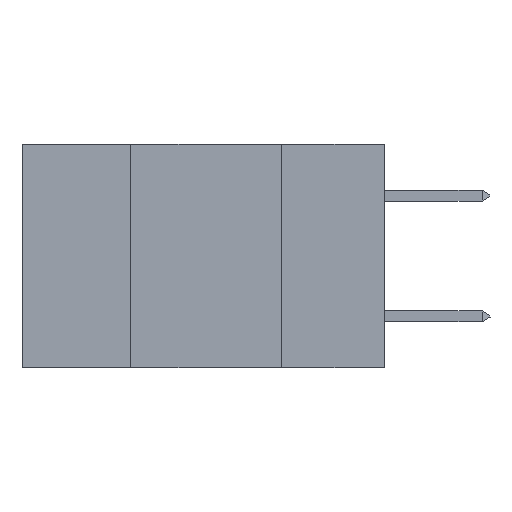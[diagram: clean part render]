
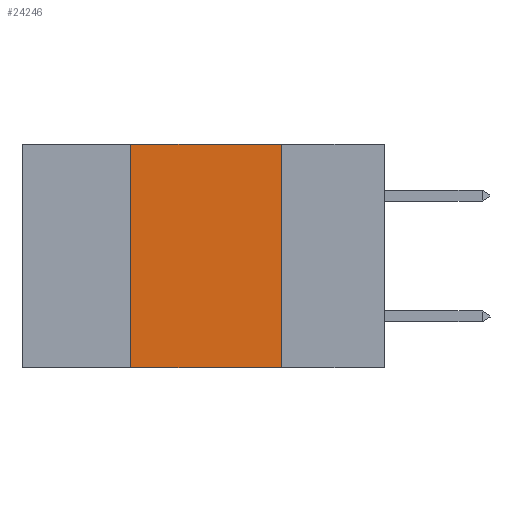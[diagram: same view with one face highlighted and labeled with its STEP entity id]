
A CAD part, left-side view. The second image highlights one B-rep face of the part: STEP entity #24246.
In plain terms, the highlighted planar face has unit normal (-1, 0, 0).
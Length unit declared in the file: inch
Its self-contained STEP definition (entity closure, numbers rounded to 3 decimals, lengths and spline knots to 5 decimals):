
#930 = ORIENTED_EDGE ( 'NONE', *, *, #37264, .F. ) ;
#1995 = DIRECTION ( 'NONE',  ( 0., 0., -1. ) ) ;
#4105 = DIRECTION ( 'NONE',  ( 0., -1., 0. ) ) ;
#5628 = CARTESIAN_POINT ( 'NONE',  ( 0., 0.17, -0.37 ) ) ;
#5698 = LINE ( 'NONE', #14263, #31536 ) ;
#7103 = EDGE_CURVE ( 'NONE', #25348, #16699, #5698, .T. ) ;
#7893 = ORIENTED_EDGE ( 'NONE', *, *, #35387, .F. ) ;
#10733 = DIRECTION ( 'NONE',  ( 0., -1., 0. ) ) ;
#10874 = CARTESIAN_POINT ( 'NONE',  ( 0., 0.17, 0. ) ) ;
#14263 = CARTESIAN_POINT ( 'NONE',  ( 0., 0.6, 0. ) ) ;
#15130 = PLANE ( 'NONE',  #18716 ) ;
#15509 = CARTESIAN_POINT ( 'NONE',  ( 0., 0.42, 0. ) ) ;
#16658 = EDGE_CURVE ( 'NONE', #29449, #40052, #29981, .T. ) ;
#16699 = VERTEX_POINT ( 'NONE', #10874 ) ;
#18544 = DIRECTION ( 'NONE',  ( 1., 0., 0. ) ) ;
#18716 = AXIS2_PLACEMENT_3D ( 'NONE', #35076, #18544, #41714 ) ;
#19047 = CARTESIAN_POINT ( 'NONE',  ( 0., 0.17, 0. ) ) ;
#19973 = LINE ( 'NONE', #19047, #27820 ) ;
#20650 = CARTESIAN_POINT ( 'NONE',  ( 0., 0.42, 0. ) ) ;
#21127 = VECTOR ( 'NONE', #10733, 39.37008 ) ;
#22186 = LINE ( 'NONE', #15509, #30266 ) ;
#24246 = ADVANCED_FACE ( 'NONE', ( #38545 ), #15130, .F. ) ;
#25348 = VERTEX_POINT ( 'NONE', #20650 ) ;
#26983 = CARTESIAN_POINT ( 'NONE',  ( 0., 0.6, -0.37 ) ) ;
#27155 = EDGE_LOOP ( 'NONE', ( #7893, #35723, #930, #37794 ) ) ;
#27820 = VECTOR ( 'NONE', #1995, 39.37008 ) ;
#28464 = CARTESIAN_POINT ( 'NONE',  ( 0., 0.42, -0.37 ) ) ;
#28834 = DIRECTION ( 'NONE',  ( 0., 0., 1. ) ) ;
#29449 = VERTEX_POINT ( 'NONE', #28464 ) ;
#29981 = LINE ( 'NONE', #26983, #21127 ) ;
#30266 = VECTOR ( 'NONE', #28834, 39.37008 ) ;
#31536 = VECTOR ( 'NONE', #4105, 39.37008 ) ;
#35076 = CARTESIAN_POINT ( 'NONE',  ( 0., 0.6, 0. ) ) ;
#35387 = EDGE_CURVE ( 'NONE', #16699, #40052, #19973, .T. ) ;
#35723 = ORIENTED_EDGE ( 'NONE', *, *, #7103, .F. ) ;
#37264 = EDGE_CURVE ( 'NONE', #29449, #25348, #22186, .T. ) ;
#37794 = ORIENTED_EDGE ( 'NONE', *, *, #16658, .T. ) ;
#38545 = FACE_OUTER_BOUND ( 'NONE', #27155, .T. ) ;
#40052 = VERTEX_POINT ( 'NONE', #5628 ) ;
#41714 = DIRECTION ( 'NONE',  ( 0., 0., -1. ) ) ;
